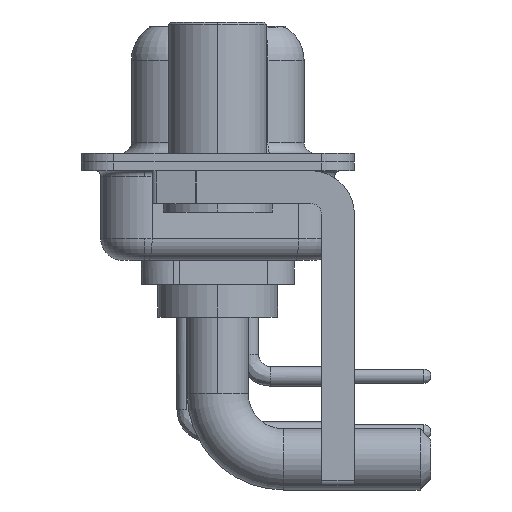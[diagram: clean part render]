
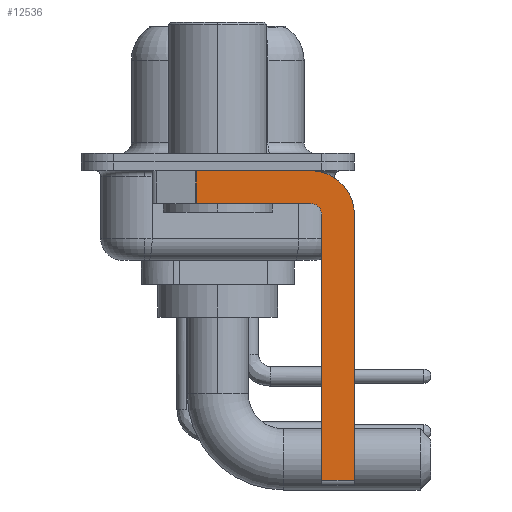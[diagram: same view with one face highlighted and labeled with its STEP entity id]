
A CAD part, left-side view. The second image highlights one B-rep face of the part: STEP entity #12536.
In plain terms, the highlighted planar face has unit normal (-1, 0, 0).
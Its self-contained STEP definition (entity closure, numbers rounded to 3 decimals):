
#103 = CARTESIAN_POINT ( 'NONE',  ( -2.9, -4.75, -14.8 ) ) ;
#794 = EDGE_CURVE ( 'NONE', #23456, #25757, #15781, .T. ) ;
#1375 = ORIENTED_EDGE ( 'NONE', *, *, #13256, .T. ) ;
#2300 = CARTESIAN_POINT ( 'NONE',  ( -2.9, 3., -0.4 ) ) ;
#2812 = PLANE ( 'NONE',  #13973 ) ;
#3130 = CARTESIAN_POINT ( 'NONE',  ( -2.9, -4.75, -2.4 ) ) ;
#3249 = ORIENTED_EDGE ( 'NONE', *, *, #18169, .T. ) ;
#3789 = CARTESIAN_POINT ( 'NONE',  ( -2.9, 0.978, -1.9 ) ) ;
#3998 = CARTESIAN_POINT ( 'NONE',  ( -2.9, 0.978, -1.9 ) ) ;
#4408 = CARTESIAN_POINT ( 'NONE',  ( -2.9, 0.978, -0.4 ) ) ;
#4475 = ORIENTED_EDGE ( 'NONE', *, *, #794, .F. ) ;
#4834 = CARTESIAN_POINT ( 'NONE',  ( -2.9, -6.25, -2.4 ) ) ;
#4912 = VECTOR ( 'NONE', #23194, 1000. ) ;
#5352 = VECTOR ( 'NONE', #17657, 1000. ) ;
#6164 = EDGE_LOOP ( 'NONE', ( #26606, #1375, #24673, #23726, #22456, #3249, #6649, #4475 ) ) ;
#6435 = CARTESIAN_POINT ( 'NONE',  ( -2.9, -4.25, -2.4 ) ) ;
#6649 = ORIENTED_EDGE ( 'NONE', *, *, #26544, .F. ) ;
#7294 = CARTESIAN_POINT ( 'NONE',  ( -2.9, -6.25, -14.55 ) ) ;
#7447 = CIRCLE ( 'NONE', #19373, 0.5 ) ;
#8560 = DIRECTION ( 'NONE',  ( 0., 0., -1. ) ) ;
#9495 = VERTEX_POINT ( 'NONE', #3130 ) ;
#9557 = VERTEX_POINT ( 'NONE', #11145 ) ;
#10831 = CARTESIAN_POINT ( 'NONE',  ( -2.9, -4.25, -1.9 ) ) ;
#11145 = CARTESIAN_POINT ( 'NONE',  ( -2.9, -4.25, -1.9 ) ) ;
#11590 = LINE ( 'NONE', #4834, #22243 ) ;
#12536 = ADVANCED_FACE ( 'NONE', ( #19817 ), #2812, .F. ) ;
#12667 = LINE ( 'NONE', #103, #21261 ) ;
#12910 = LINE ( 'NONE', #10831, #22420 ) ;
#13256 = EDGE_CURVE ( 'NONE', #16693, #15543, #19079, .T. ) ;
#13258 = DIRECTION ( 'NONE',  ( 0., 0., -1. ) ) ;
#13669 = EDGE_CURVE ( 'NONE', #9557, #15543, #12910, .T. ) ;
#13973 = AXIS2_PLACEMENT_3D ( 'NONE', #15381, #21904, #24110 ) ;
#14302 = EDGE_CURVE ( 'NONE', #9495, #9557, #7447, .T. ) ;
#14745 = DIRECTION ( 'NONE',  ( 0., 0., 1. ) ) ;
#15381 = CARTESIAN_POINT ( 'NONE',  ( -2.9, -4.25, -2.4 ) ) ;
#15499 = CARTESIAN_POINT ( 'NONE',  ( -2.9, -4.25, -2.4 ) ) ;
#15543 = VERTEX_POINT ( 'NONE', #3789 ) ;
#15764 = VECTOR ( 'NONE', #8560, 1000. ) ;
#15781 = CIRCLE ( 'NONE', #16212, 2. ) ;
#16212 = AXIS2_PLACEMENT_3D ( 'NONE', #6435, #25372, #16787 ) ;
#16693 = VERTEX_POINT ( 'NONE', #4408 ) ;
#16787 = DIRECTION ( 'NONE',  ( 0., 0., -1. ) ) ;
#17295 = DIRECTION ( 'NONE',  ( 0., 0., 1. ) ) ;
#17657 = DIRECTION ( 'NONE',  ( 0., -1., 0. ) ) ;
#17933 = LINE ( 'NONE', #24049, #5352 ) ;
#18169 = EDGE_CURVE ( 'NONE', #18464, #21359, #17933, .T. ) ;
#18397 = EDGE_CURVE ( 'NONE', #16693, #23456, #19312, .T. ) ;
#18464 = VERTEX_POINT ( 'NONE', #23331 ) ;
#19079 = LINE ( 'NONE', #3998, #15764 ) ;
#19312 = LINE ( 'NONE', #2300, #4912 ) ;
#19373 = AXIS2_PLACEMENT_3D ( 'NONE', #15499, #23546, #17295 ) ;
#19817 = FACE_OUTER_BOUND ( 'NONE', #6164, .T. ) ;
#21261 = VECTOR ( 'NONE', #14745, 1000. ) ;
#21359 = VERTEX_POINT ( 'NONE', #7294 ) ;
#21904 = DIRECTION ( 'NONE',  ( 1., 0., 0. ) ) ;
#22243 = VECTOR ( 'NONE', #13258, 1000. ) ;
#22420 = VECTOR ( 'NONE', #23300, 1000. ) ;
#22456 = ORIENTED_EDGE ( 'NONE', *, *, #24625, .F. ) ;
#23194 = DIRECTION ( 'NONE',  ( 0., -1., 0. ) ) ;
#23300 = DIRECTION ( 'NONE',  ( 0., 1., 0. ) ) ;
#23331 = CARTESIAN_POINT ( 'NONE',  ( -2.9, -4.75, -14.55 ) ) ;
#23456 = VERTEX_POINT ( 'NONE', #25593 ) ;
#23546 = DIRECTION ( 'NONE',  ( -1., 0., 0. ) ) ;
#23726 = ORIENTED_EDGE ( 'NONE', *, *, #14302, .F. ) ;
#24049 = CARTESIAN_POINT ( 'NONE',  ( -2.9, -4.25, -14.55 ) ) ;
#24110 = DIRECTION ( 'NONE',  ( 0., 0., -1. ) ) ;
#24573 = CARTESIAN_POINT ( 'NONE',  ( -2.9, -6.25, -2.4 ) ) ;
#24625 = EDGE_CURVE ( 'NONE', #18464, #9495, #12667, .T. ) ;
#24673 = ORIENTED_EDGE ( 'NONE', *, *, #13669, .F. ) ;
#25372 = DIRECTION ( 'NONE',  ( 1., 0., 0. ) ) ;
#25593 = CARTESIAN_POINT ( 'NONE',  ( -2.9, -4.25, -0.4 ) ) ;
#25757 = VERTEX_POINT ( 'NONE', #24573 ) ;
#26544 = EDGE_CURVE ( 'NONE', #25757, #21359, #11590, .T. ) ;
#26606 = ORIENTED_EDGE ( 'NONE', *, *, #18397, .F. ) ;
